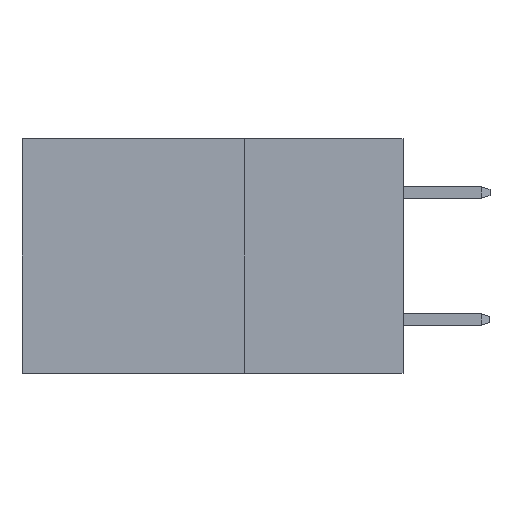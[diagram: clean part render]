
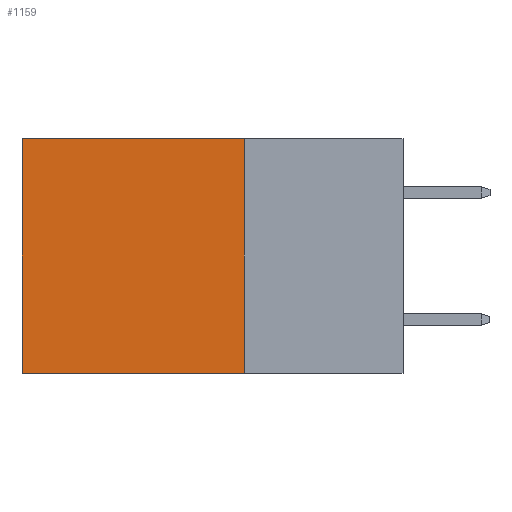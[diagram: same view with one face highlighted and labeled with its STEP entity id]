
A CAD part, left-side view. The second image highlights one B-rep face of the part: STEP entity #1159.
In plain terms, the highlighted planar face has unit normal (-1, 0, 0).
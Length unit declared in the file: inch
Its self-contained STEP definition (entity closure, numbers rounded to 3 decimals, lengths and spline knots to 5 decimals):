
#826 = DIRECTION ( 'NONE',  ( 0., 1., 0. ) ) ;
#888 = CARTESIAN_POINT ( 'NONE',  ( 0.2875, 0.25, -0.37 ) ) ;
#1159 = ADVANCED_FACE ( 'NONE', ( #8164 ), #7004, .F. ) ;
#1475 = VECTOR ( 'NONE', #826, 39.37008 ) ;
#1881 = CARTESIAN_POINT ( 'NONE',  ( 0.2875, 0.25, -0.37 ) ) ;
#2065 = EDGE_CURVE ( 'NONE', #9234, #5270, #9096, .T. ) ;
#2438 = ORIENTED_EDGE ( 'NONE', *, *, #2065, .F. ) ;
#2541 = DIRECTION ( 'NONE',  ( 1., 0., 0. ) ) ;
#2650 = ORIENTED_EDGE ( 'NONE', *, *, #7556, .F. ) ;
#3649 = EDGE_LOOP ( 'NONE', ( #9950, #2650, #2438, #7657 ) ) ;
#3755 = DIRECTION ( 'NONE',  ( 0., 0., -1. ) ) ;
#4193 = DIRECTION ( 'NONE',  ( 0., 0., -1. ) ) ;
#4632 = CARTESIAN_POINT ( 'NONE',  ( 0.2875, 0.25, 0. ) ) ;
#5247 = CARTESIAN_POINT ( 'NONE',  ( 0.2875, 0.6, 0. ) ) ;
#5270 = VERTEX_POINT ( 'NONE', #1881 ) ;
#6249 = DIRECTION ( 'NONE',  ( 0., 0., -1. ) ) ;
#6479 = LINE ( 'NONE', #4632, #11328 ) ;
#7004 = PLANE ( 'NONE',  #11757 ) ;
#7556 = EDGE_CURVE ( 'NONE', #5270, #9381, #8302, .T. ) ;
#7657 = ORIENTED_EDGE ( 'NONE', *, *, #8734, .T. ) ;
#8164 = FACE_OUTER_BOUND ( 'NONE', #3649, .T. ) ;
#8302 = LINE ( 'NONE', #888, #1475 ) ;
#8393 = DIRECTION ( 'NONE',  ( 0., 1., 0. ) ) ;
#8602 = VECTOR ( 'NONE', #3755, 39.37008 ) ;
#8734 = EDGE_CURVE ( 'NONE', #9234, #11010, #6479, .T. ) ;
#9033 = CARTESIAN_POINT ( 'NONE',  ( 0.2875, 0.25, 0. ) ) ;
#9096 = LINE ( 'NONE', #9033, #10781 ) ;
#9234 = VERTEX_POINT ( 'NONE', #11594 ) ;
#9381 = VERTEX_POINT ( 'NONE', #11056 ) ;
#9864 = CARTESIAN_POINT ( 'NONE',  ( 0.2875, 0.6, 0. ) ) ;
#9923 = LINE ( 'NONE', #5247, #8602 ) ;
#9950 = ORIENTED_EDGE ( 'NONE', *, *, #10449, .T. ) ;
#10449 = EDGE_CURVE ( 'NONE', #11010, #9381, #9923, .T. ) ;
#10781 = VECTOR ( 'NONE', #4193, 39.37008 ) ;
#11010 = VERTEX_POINT ( 'NONE', #9864 ) ;
#11056 = CARTESIAN_POINT ( 'NONE',  ( 0.2875, 0.6, -0.37 ) ) ;
#11328 = VECTOR ( 'NONE', #8393, 39.37008 ) ;
#11594 = CARTESIAN_POINT ( 'NONE',  ( 0.2875, 0.25, 0. ) ) ;
#11757 = AXIS2_PLACEMENT_3D ( 'NONE', #11914, #2541, #6249 ) ;
#11914 = CARTESIAN_POINT ( 'NONE',  ( 0.2875, 0.25, 0. ) ) ;
